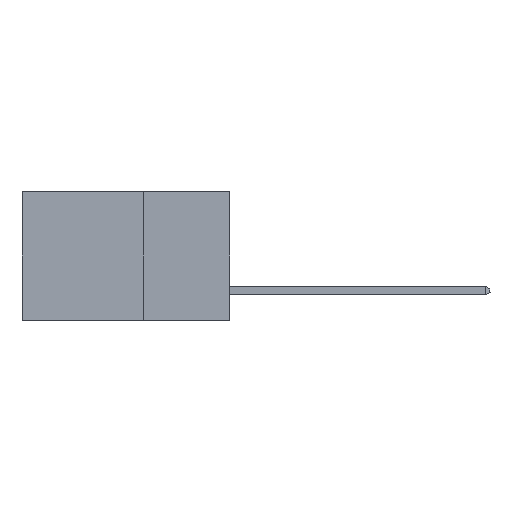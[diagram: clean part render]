
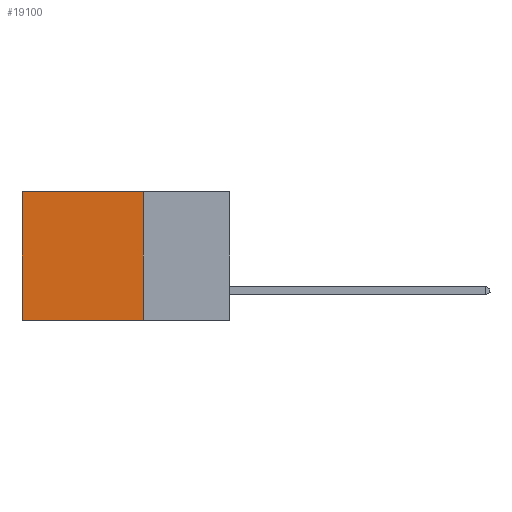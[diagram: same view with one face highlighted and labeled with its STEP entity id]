
A CAD part, left-side view. The second image highlights one B-rep face of the part: STEP entity #19100.
In plain terms, the highlighted planar face has unit normal (-1, 0, 0).
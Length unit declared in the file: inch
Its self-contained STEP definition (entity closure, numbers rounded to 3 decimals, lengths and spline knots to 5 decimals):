
#315 = DIRECTION ( 'NONE',  ( 0., 1., 0. ) ) ;
#1753 = VECTOR ( 'NONE', #10183, 39.37008 ) ;
#2048 = CARTESIAN_POINT ( 'NONE',  ( 0.298, 0.25, 0. ) ) ;
#2641 = FACE_OUTER_BOUND ( 'NONE', #21879, .T. ) ;
#3207 = CARTESIAN_POINT ( 'NONE',  ( 0.298, 0.6, 0. ) ) ;
#4503 = CARTESIAN_POINT ( 'NONE',  ( 0.298, 0.25, -0.37 ) ) ;
#4584 = PLANE ( 'NONE',  #15741 ) ;
#4628 = VERTEX_POINT ( 'NONE', #9863 ) ;
#5983 = EDGE_CURVE ( 'NONE', #23931, #4628, #15523, .T. ) ;
#8086 = DIRECTION ( 'NONE',  ( 0., 1., 0. ) ) ;
#9671 = LINE ( 'NONE', #12778, #1753 ) ;
#9863 = CARTESIAN_POINT ( 'NONE',  ( 0.298, 0.6, 0. ) ) ;
#10183 = DIRECTION ( 'NONE',  ( 0., 0., -1. ) ) ;
#10945 = ORIENTED_EDGE ( 'NONE', *, *, #25364, .T. ) ;
#11067 = VECTOR ( 'NONE', #22382, 39.37008 ) ;
#11583 = DIRECTION ( 'NONE',  ( 1., 0., 0. ) ) ;
#12151 = VECTOR ( 'NONE', #8086, 39.37008 ) ;
#12203 = CARTESIAN_POINT ( 'NONE',  ( 0.298, 0.6, -0.37 ) ) ;
#12778 = CARTESIAN_POINT ( 'NONE',  ( 0.298, 0.25, 0. ) ) ;
#15074 = LINE ( 'NONE', #19360, #24096 ) ;
#15237 = CARTESIAN_POINT ( 'NONE',  ( 0.298, 0.25, 0. ) ) ;
#15523 = LINE ( 'NONE', #15237, #12151 ) ;
#15741 = AXIS2_PLACEMENT_3D ( 'NONE', #19119, #11583, #28489 ) ;
#15984 = VERTEX_POINT ( 'NONE', #4503 ) ;
#16354 = EDGE_CURVE ( 'NONE', #23931, #15984, #9671, .T. ) ;
#17810 = LINE ( 'NONE', #3207, #11067 ) ;
#19100 = ADVANCED_FACE ( 'NONE', ( #2641 ), #4584, .F. ) ;
#19119 = CARTESIAN_POINT ( 'NONE',  ( 0.298, 0.25, 0. ) ) ;
#19360 = CARTESIAN_POINT ( 'NONE',  ( 0.298, 0.25, -0.37 ) ) ;
#21806 = ORIENTED_EDGE ( 'NONE', *, *, #16354, .F. ) ;
#21879 = EDGE_LOOP ( 'NONE', ( #10945, #24698, #21806, #30545 ) ) ;
#22382 = DIRECTION ( 'NONE',  ( 0., 0., -1. ) ) ;
#23931 = VERTEX_POINT ( 'NONE', #2048 ) ;
#24096 = VECTOR ( 'NONE', #315, 39.37008 ) ;
#24698 = ORIENTED_EDGE ( 'NONE', *, *, #26599, .F. ) ;
#25364 = EDGE_CURVE ( 'NONE', #4628, #28089, #17810, .T. ) ;
#26599 = EDGE_CURVE ( 'NONE', #15984, #28089, #15074, .T. ) ;
#28089 = VERTEX_POINT ( 'NONE', #12203 ) ;
#28489 = DIRECTION ( 'NONE',  ( 0., 0., -1. ) ) ;
#30545 = ORIENTED_EDGE ( 'NONE', *, *, #5983, .T. ) ;
